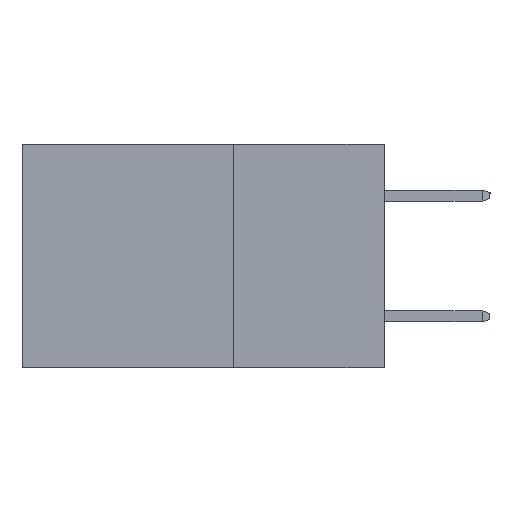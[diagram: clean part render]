
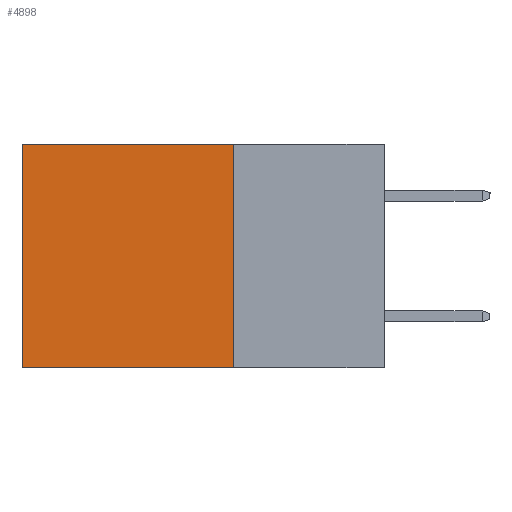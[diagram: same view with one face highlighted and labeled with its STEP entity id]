
A CAD part, left-side view. The second image highlights one B-rep face of the part: STEP entity #4898.
In plain terms, the highlighted planar face has unit normal (-1, 0, 0).
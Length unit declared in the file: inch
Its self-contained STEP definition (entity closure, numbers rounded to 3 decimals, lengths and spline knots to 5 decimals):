
#244 = VERTEX_POINT ( 'NONE', #6079 ) ;
#594 = ORIENTED_EDGE ( 'NONE', *, *, #6150, .F. ) ;
#741 = VERTEX_POINT ( 'NONE', #5328 ) ;
#754 = DIRECTION ( 'NONE',  ( 0., 0., -1. ) ) ;
#2408 = ORIENTED_EDGE ( 'NONE', *, *, #13530, .T. ) ;
#2500 = DIRECTION ( 'NONE',  ( 0., 0., -1. ) ) ;
#2536 = LINE ( 'NONE', #10412, #3519 ) ;
#2761 = VERTEX_POINT ( 'NONE', #12999 ) ;
#3430 = ORIENTED_EDGE ( 'NONE', *, *, #10484, .T. ) ;
#3519 = VECTOR ( 'NONE', #754, 39.37008 ) ;
#3866 = LINE ( 'NONE', #7985, #9477 ) ;
#4801 = DIRECTION ( 'NONE',  ( 1., 0., 0. ) ) ;
#4898 = ADVANCED_FACE ( 'NONE', ( #8012 ), #9065, .F. ) ;
#4906 = EDGE_LOOP ( 'NONE', ( #2408, #8945, #594, #3430 ) ) ;
#5328 = CARTESIAN_POINT ( 'NONE',  ( 0.2615, 0.6, -0.37 ) ) ;
#6079 = CARTESIAN_POINT ( 'NONE',  ( 0.2615, 0.25, 0. ) ) ;
#6150 = EDGE_CURVE ( 'NONE', #244, #6731, #12219, .T. ) ;
#6519 = CARTESIAN_POINT ( 'NONE',  ( 0.2615, 0.25, -0.37 ) ) ;
#6731 = VERTEX_POINT ( 'NONE', #8273 ) ;
#7031 = AXIS2_PLACEMENT_3D ( 'NONE', #10187, #4801, #9129 ) ;
#7452 = DIRECTION ( 'NONE',  ( 0., 1., 0. ) ) ;
#7770 = VECTOR ( 'NONE', #7452, 39.37008 ) ;
#7985 = CARTESIAN_POINT ( 'NONE',  ( 0.2615, 0.25, 0. ) ) ;
#8012 = FACE_OUTER_BOUND ( 'NONE', #4906, .T. ) ;
#8083 = EDGE_CURVE ( 'NONE', #6731, #741, #12662, .T. ) ;
#8273 = CARTESIAN_POINT ( 'NONE',  ( 0.2615, 0.25, -0.37 ) ) ;
#8945 = ORIENTED_EDGE ( 'NONE', *, *, #8083, .F. ) ;
#9065 = PLANE ( 'NONE',  #7031 ) ;
#9129 = DIRECTION ( 'NONE',  ( 0., 0., -1. ) ) ;
#9131 = CARTESIAN_POINT ( 'NONE',  ( 0.2615, 0.25, -0.37 ) ) ;
#9477 = VECTOR ( 'NONE', #13461, 39.37008 ) ;
#10187 = CARTESIAN_POINT ( 'NONE',  ( 0.2615, 0.25, -0.37 ) ) ;
#10209 = VECTOR ( 'NONE', #2500, 39.37008 ) ;
#10412 = CARTESIAN_POINT ( 'NONE',  ( 0.2615, 0.6, -0.37 ) ) ;
#10484 = EDGE_CURVE ( 'NONE', #244, #2761, #3866, .T. ) ;
#12219 = LINE ( 'NONE', #9131, #10209 ) ;
#12662 = LINE ( 'NONE', #6519, #7770 ) ;
#12999 = CARTESIAN_POINT ( 'NONE',  ( 0.2615, 0.6, 0. ) ) ;
#13461 = DIRECTION ( 'NONE',  ( 0., 1., 0. ) ) ;
#13530 = EDGE_CURVE ( 'NONE', #2761, #741, #2536, .T. ) ;
